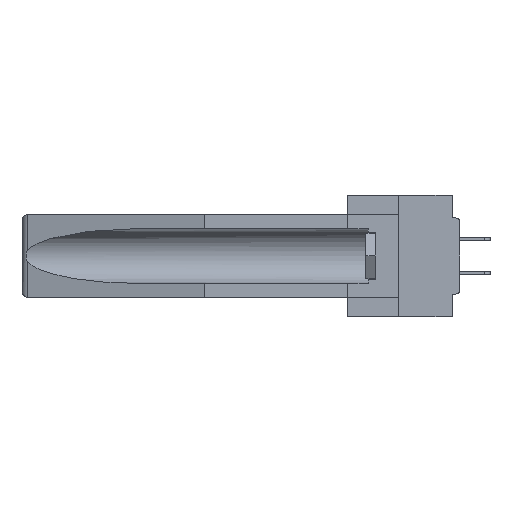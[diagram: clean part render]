
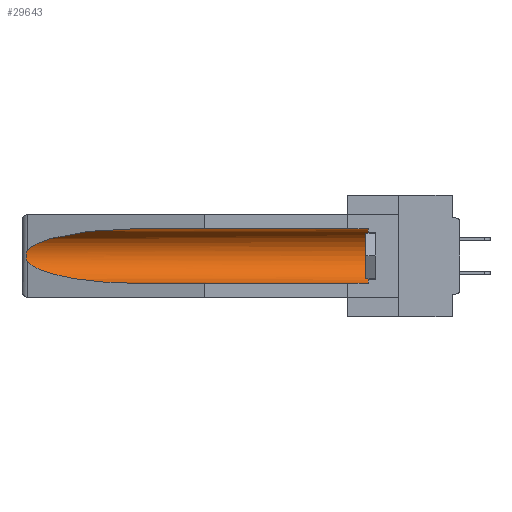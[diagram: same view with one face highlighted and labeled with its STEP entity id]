
A CAD part, left-side view. The second image highlights one B-rep face of the part: STEP entity #29643.
In plain terms, the highlighted cylindrical face has radius 2.857 mm (diameter 5.715 mm), a partial arc.
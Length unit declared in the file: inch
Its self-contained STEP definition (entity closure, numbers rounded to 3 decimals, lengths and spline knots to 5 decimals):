
#112 = EDGE_CURVE ( 'NONE', #34383, #23751, #28636, .T. ) ;
#791 = CARTESIAN_POINT ( 'NONE',  ( 0.21114, 1.30732, -0.284 ) ) ;
#939 = CARTESIAN_POINT ( 'NONE',  ( 0.26537, 1.52718, -0.14972 ) ) ;
#2223 = CARTESIAN_POINT ( 'NONE',  ( 0.2673, 1.5327, -0.16383 ) ) ;
#3691 = EDGE_CURVE ( 'NONE', #7236, #23751, #12574, .T. ) ;
#3695 = LINE ( 'NONE', #36872, #18046 ) ;
#6629 = CARTESIAN_POINT ( 'NONE',  ( 0.155, 1.07973, -0.059 ) ) ;
#7236 = VERTEX_POINT ( 'NONE', #24654 ) ;
#7487 = EDGE_CURVE ( 'NONE', #35298, #7236, #34231, .T. ) ;
#7748 = CARTESIAN_POINT ( 'NONE',  ( 0.26655, 1.53094, -0.18657 ) ) ;
#8582 = CARTESIAN_POINT ( 'NONE',  ( 0.26537, 1.52718, -0.14972 ) ) ;
#8946 = CARTESIAN_POINT ( 'NONE',  ( 0.155, 1.07973, -0.284 ) ) ;
#9666 = ORIENTED_EDGE ( 'NONE', *, *, #7487, .T. ) ;
#10531 = CARTESIAN_POINT ( 'NONE',  ( 0.26537, 1.52718, -0.19328 ) ) ;
#10935 = DIRECTION ( 'NONE',  ( 0., 0., 1. ) ) ;
#11568 = DIRECTION ( 'NONE',  ( 0., -1., 0. ) ) ;
#11782 = ORIENTED_EDGE ( 'NONE', *, *, #3691, .T. ) ;
#12574 =( BOUNDED_CURVE ( )  B_SPLINE_CURVE ( 3, ( #32316, #29167, #791, #8946 ),
 .UNSPECIFIED., .F., .T. ) 
 B_SPLINE_CURVE_WITH_KNOTS ( ( 4, 4 ),
 ( 0.1948, 1.5708 ),
 .UNSPECIFIED. ) 
 CURVE ( )  GEOMETRIC_REPRESENTATION_ITEM ( )  RATIONAL_B_SPLINE_CURVE ( ( 1., 0.848, 0.848, 1. ) ) 
 REPRESENTATION_ITEM ( '' )  );
#13274 = CARTESIAN_POINT ( 'NONE',  ( 0.155, 1.07973, -0.284 ) ) ;
#13657 = ORIENTED_EDGE ( 'NONE', *, *, #21024, .T. ) ;
#14461 = DIRECTION ( 'NONE',  ( 0., 0., 1. ) ) ;
#14981 = CARTESIAN_POINT ( 'NONE',  ( 0.155, 0.126, -0.1715 ) ) ;
#16040 = FACE_OUTER_BOUND ( 'NONE', #22747, .T. ) ;
#16680 = EDGE_CURVE ( 'NONE', #34383, #28307, #19744, .T. ) ;
#16729 = CARTESIAN_POINT ( 'NONE',  ( 0.155, -0.30754, -0.1715 ) ) ;
#16752 = DIRECTION ( 'NONE',  ( 0., 1., 0. ) ) ;
#17834 = CYLINDRICAL_SURFACE ( 'NONE', #33220, 0.1125 ) ;
#18046 = VECTOR ( 'NONE', #16752, 39.37008 ) ;
#18380 = CARTESIAN_POINT ( 'NONE',  ( 0.25451, 1.48313, -0.09465 ) ) ;
#18716 = DIRECTION ( 'NONE',  ( 0., 1., 0. ) ) ;
#19185 = CARTESIAN_POINT ( 'NONE',  ( 0.26597, 1.52961, -0.15275 ) ) ;
#19744 = CIRCLE ( 'NONE', #21983, 0.1125 ) ;
#21019 = VECTOR ( 'NONE', #18716, 39.37008 ) ;
#21024 = EDGE_CURVE ( 'NONE', #32788, #35298, #23161, .T. ) ;
#21699 = ORIENTED_EDGE ( 'NONE', *, *, #33070, .T. ) ;
#21958 = CARTESIAN_POINT ( 'NONE',  ( 0.26654, 1.53092, -0.15636 ) ) ;
#21983 = AXIS2_PLACEMENT_3D ( 'NONE', #14981, #11568, #14461 ) ;
#22198 = CARTESIAN_POINT ( 'NONE',  ( 0.2675, 1.53308, -0.17534 ) ) ;
#22373 = CARTESIAN_POINT ( 'NONE',  ( 0.155, 0.126, -0.284 ) ) ;
#22747 = EDGE_LOOP ( 'NONE', ( #13657, #9666, #11782, #33278, #32594, #21699 ) ) ;
#23161 =( BOUNDED_CURVE ( )  B_SPLINE_CURVE ( 3, ( #23286, #32455, #18380, #939 ),
 .UNSPECIFIED., .F., .F. ) 
 B_SPLINE_CURVE_WITH_KNOTS ( ( 4, 4 ),
 ( 4.71239, 6.08839 ),
 .UNSPECIFIED. ) 
 CURVE ( )  GEOMETRIC_REPRESENTATION_ITEM ( )  RATIONAL_B_SPLINE_CURVE ( ( 1., 0.848, 0.848, 1. ) ) 
 REPRESENTATION_ITEM ( '' )  );
#23286 = CARTESIAN_POINT ( 'NONE',  ( 0.155, 1.07973, -0.059 ) ) ;
#23751 = VERTEX_POINT ( 'NONE', #13274 ) ;
#24362 = CARTESIAN_POINT ( 'NONE',  ( 0.155, -0.30754, -0.284 ) ) ;
#24654 = CARTESIAN_POINT ( 'NONE',  ( 0.26537, 1.52718, -0.19328 ) ) ;
#25257 = DIRECTION ( 'NONE',  ( 0., 1., 0. ) ) ;
#27720 = CARTESIAN_POINT ( 'NONE',  ( 0.26597, 1.5296, -0.19026 ) ) ;
#28307 = VERTEX_POINT ( 'NONE', #29220 ) ;
#28636 = LINE ( 'NONE', #24362, #21019 ) ;
#29167 = CARTESIAN_POINT ( 'NONE',  ( 0.25451, 1.48313, -0.24835 ) ) ;
#29220 = CARTESIAN_POINT ( 'NONE',  ( 0.155, 0.126, -0.059 ) ) ;
#29643 = ADVANCED_FACE ( 'NONE', ( #16040 ), #17834, .F. ) ;
#30868 = CARTESIAN_POINT ( 'NONE',  ( 0.2673, 1.53269, -0.17917 ) ) ;
#32316 = CARTESIAN_POINT ( 'NONE',  ( 0.26537, 1.52718, -0.19328 ) ) ;
#32455 = CARTESIAN_POINT ( 'NONE',  ( 0.21114, 1.30732, -0.059 ) ) ;
#32594 = ORIENTED_EDGE ( 'NONE', *, *, #16680, .T. ) ;
#32788 = VERTEX_POINT ( 'NONE', #6629 ) ;
#33070 = EDGE_CURVE ( 'NONE', #28307, #32788, #3695, .T. ) ;
#33220 = AXIS2_PLACEMENT_3D ( 'NONE', #16729, #25257, #10935 ) ;
#33278 = ORIENTED_EDGE ( 'NONE', *, *, #112, .F. ) ;
#33875 = CARTESIAN_POINT ( 'NONE',  ( 0.2675, 1.53308, -0.16763 ) ) ;
#34231 = B_SPLINE_CURVE_WITH_KNOTS ( 'NONE', 3,
 ( #36425, #19185, #21958, #2223, #33875, #22198, #30868, #7748, #27720, #10531 ),
 .UNSPECIFIED., .F., .F.,
 ( 4, 2, 2, 2, 4 ),
 ( 0., 0.00029, 0.00058, 0.00087, 0.00117 ),
 .UNSPECIFIED. ) ;
#34383 = VERTEX_POINT ( 'NONE', #22373 ) ;
#35298 = VERTEX_POINT ( 'NONE', #8582 ) ;
#36425 = CARTESIAN_POINT ( 'NONE',  ( 0.26537, 1.52718, -0.14972 ) ) ;
#36872 = CARTESIAN_POINT ( 'NONE',  ( 0.155, -0.30754, -0.059 ) ) ;
